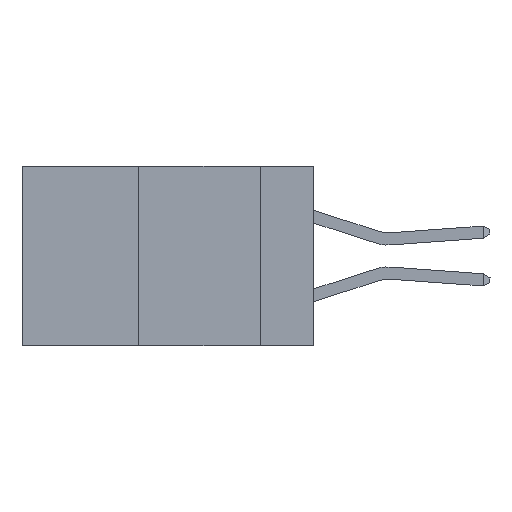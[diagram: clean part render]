
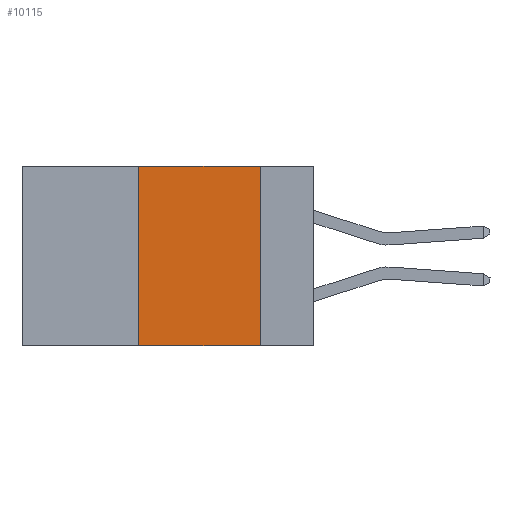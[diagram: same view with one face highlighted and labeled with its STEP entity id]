
A CAD part, left-side view. The second image highlights one B-rep face of the part: STEP entity #10115.
In plain terms, the highlighted planar face has unit normal (-1, 0, 0).
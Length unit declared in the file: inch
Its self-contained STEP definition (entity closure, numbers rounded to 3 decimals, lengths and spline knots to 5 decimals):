
#109 = CARTESIAN_POINT ( 'NONE',  ( 0., 0.36, 0. ) ) ;
#307 = VECTOR ( 'NONE', #3801, 39.37008 ) ;
#605 = VECTOR ( 'NONE', #4732, 39.37008 ) ;
#1803 = EDGE_CURVE ( 'NONE', #2906, #11243, #7424, .T. ) ;
#2286 = VECTOR ( 'NONE', #3104, 39.37008 ) ;
#2395 = DIRECTION ( 'NONE',  ( 1., 0., 0. ) ) ;
#2906 = VERTEX_POINT ( 'NONE', #109 ) ;
#3104 = DIRECTION ( 'NONE',  ( 0., -1., 0. ) ) ;
#3801 = DIRECTION ( 'NONE',  ( 0., 0., -1. ) ) ;
#3809 = AXIS2_PLACEMENT_3D ( 'NONE', #8749, #2395, #10749 ) ;
#4049 = ORIENTED_EDGE ( 'NONE', *, *, #4355, .F. ) ;
#4355 = EDGE_CURVE ( 'NONE', #11243, #7551, #5931, .T. ) ;
#4732 = DIRECTION ( 'NONE',  ( 0., 0., 1. ) ) ;
#5265 = CARTESIAN_POINT ( 'NONE',  ( 0., 0.11, 0. ) ) ;
#5462 = FACE_OUTER_BOUND ( 'NONE', #5899, .T. ) ;
#5899 = EDGE_LOOP ( 'NONE', ( #4049, #8047, #10199, #6394 ) ) ;
#5931 = LINE ( 'NONE', #9000, #307 ) ;
#6046 = DIRECTION ( 'NONE',  ( 0., -1., 0. ) ) ;
#6394 = ORIENTED_EDGE ( 'NONE', *, *, #11911, .T. ) ;
#7284 = CARTESIAN_POINT ( 'NONE',  ( 0., 0.36, -0.37 ) ) ;
#7424 = LINE ( 'NONE', #10229, #13568 ) ;
#7551 = VERTEX_POINT ( 'NONE', #9424 ) ;
#8047 = ORIENTED_EDGE ( 'NONE', *, *, #1803, .F. ) ;
#8108 = LINE ( 'NONE', #9146, #605 ) ;
#8344 = VERTEX_POINT ( 'NONE', #7284 ) ;
#8700 = PLANE ( 'NONE',  #3809 ) ;
#8749 = CARTESIAN_POINT ( 'NONE',  ( 0., 0.6, 0. ) ) ;
#9000 = CARTESIAN_POINT ( 'NONE',  ( 0., 0.11, 0. ) ) ;
#9146 = CARTESIAN_POINT ( 'NONE',  ( 0., 0.36, 0. ) ) ;
#9424 = CARTESIAN_POINT ( 'NONE',  ( 0., 0.11, -0.37 ) ) ;
#9659 = CARTESIAN_POINT ( 'NONE',  ( 0., 0.6, -0.37 ) ) ;
#10115 = ADVANCED_FACE ( 'NONE', ( #5462 ), #8700, .F. ) ;
#10199 = ORIENTED_EDGE ( 'NONE', *, *, #11093, .F. ) ;
#10229 = CARTESIAN_POINT ( 'NONE',  ( 0., 0.6, 0. ) ) ;
#10400 = LINE ( 'NONE', #9659, #2286 ) ;
#10749 = DIRECTION ( 'NONE',  ( 0., 0., -1. ) ) ;
#11093 = EDGE_CURVE ( 'NONE', #8344, #2906, #8108, .T. ) ;
#11243 = VERTEX_POINT ( 'NONE', #5265 ) ;
#11911 = EDGE_CURVE ( 'NONE', #8344, #7551, #10400, .T. ) ;
#13568 = VECTOR ( 'NONE', #6046, 39.37008 ) ;
